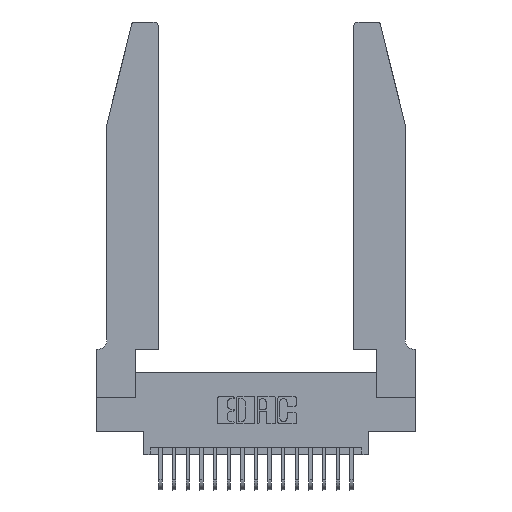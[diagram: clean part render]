
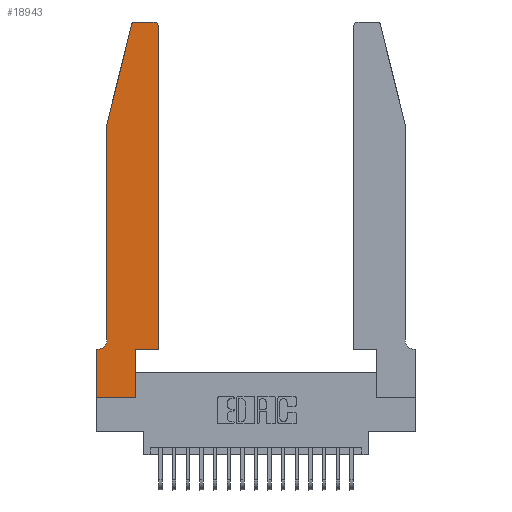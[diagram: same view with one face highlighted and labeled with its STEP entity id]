
A CAD part, top view. The second image highlights one B-rep face of the part: STEP entity #18943.
In plain terms, the highlighted planar face has unit normal (0, 0, 1).
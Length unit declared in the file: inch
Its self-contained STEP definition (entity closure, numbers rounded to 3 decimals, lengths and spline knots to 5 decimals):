
#37 = AXIS2_PLACEMENT_3D ( 'NONE', #13220, #3085, #14944 ) ;
#195 = ORIENTED_EDGE ( 'NONE', *, *, #10193, .T. ) ;
#387 = ORIENTED_EDGE ( 'NONE', *, *, #18961, .T. ) ;
#480 = CARTESIAN_POINT ( 'NONE',  ( 0.284, 2.75, 0.37 ) ) ;
#487 = DIRECTION ( 'NONE',  ( 1., 0., 0. ) ) ;
#775 = DIRECTION ( 'NONE',  ( 1., 0., 0. ) ) ;
#1053 = VERTEX_POINT ( 'NONE', #480 ) ;
#1071 = CARTESIAN_POINT ( 'NONE',  ( 0.4505, 0.35, 0.37 ) ) ;
#1951 = LINE ( 'NONE', #21206, #5494 ) ;
#1986 = VECTOR ( 'NONE', #10665, 39.37008 ) ;
#2110 = EDGE_LOOP ( 'NONE', ( #387, #195, #18907, #20903, #11278, #15937, #6031, #13395, #3044, #10007, #4897, #3687 ) ) ;
#2429 = VECTOR ( 'NONE', #4687, 39.37008 ) ;
#2494 = EDGE_CURVE ( 'NONE', #15002, #19544, #7154, .T. ) ;
#2525 = VERTEX_POINT ( 'NONE', #14175 ) ;
#2544 = CARTESIAN_POINT ( 'NONE',  ( 0., 0.35, 0.37 ) ) ;
#2557 = DIRECTION ( 'NONE',  ( 0., 0., 1. ) ) ;
#2631 = DIRECTION ( 'NONE',  ( -1., 0., 0. ) ) ;
#2947 = CARTESIAN_POINT ( 'NONE',  ( 0.0755, 0.35, 0.37 ) ) ;
#3044 = ORIENTED_EDGE ( 'NONE', *, *, #2494, .T. ) ;
#3047 = CARTESIAN_POINT ( 'NONE',  ( 0.0055, 0.35, 0.37 ) ) ;
#3085 = DIRECTION ( 'NONE',  ( 0., 0., -1. ) ) ;
#3164 = AXIS2_PLACEMENT_3D ( 'NONE', #20830, #10757, #487 ) ;
#3174 = CARTESIAN_POINT ( 'NONE',  ( 0.0755, 2., 0.37 ) ) ;
#3519 = EDGE_CURVE ( 'NONE', #15078, #15002, #1951, .T. ) ;
#3687 = ORIENTED_EDGE ( 'NONE', *, *, #5299, .T. ) ;
#4062 = VERTEX_POINT ( 'NONE', #18495 ) ;
#4203 = DIRECTION ( 'NONE',  ( 0., 1., 0. ) ) ;
#4465 = CARTESIAN_POINT ( 'NONE',  ( 0.4205, 2.75, 0.37 ) ) ;
#4687 = DIRECTION ( 'NONE',  ( -1., 0., 0. ) ) ;
#4728 = EDGE_CURVE ( 'NONE', #10207, #15078, #14430, .T. ) ;
#4827 = AXIS2_PLACEMENT_3D ( 'NONE', #21090, #11024, #775 ) ;
#4830 = CIRCLE ( 'NONE', #37, 0.07 ) ;
#4897 = ORIENTED_EDGE ( 'NONE', *, *, #21075, .T. ) ;
#4906 = LINE ( 'NONE', #12228, #13327 ) ;
#5299 = EDGE_CURVE ( 'NONE', #4062, #16967, #16251, .T. ) ;
#5494 = VECTOR ( 'NONE', #21252, 39.37008 ) ;
#5569 = EDGE_CURVE ( 'NONE', #7996, #10207, #15981, .T. ) ;
#6031 = ORIENTED_EDGE ( 'NONE', *, *, #4728, .T. ) ;
#6764 = DIRECTION ( 'NONE',  ( 0., -1., 0. ) ) ;
#6854 = VERTEX_POINT ( 'NONE', #18290 ) ;
#7154 = LINE ( 'NONE', #19578, #1986 ) ;
#7356 = LINE ( 'NONE', #9435, #20232 ) ;
#7603 = DIRECTION ( 'NONE',  ( -0.239, -0.971, 0. ) ) ;
#7996 = VERTEX_POINT ( 'NONE', #3047 ) ;
#9435 = CARTESIAN_POINT ( 'NONE',  ( 0.2605, 2.75, 0.37 ) ) ;
#9469 = CARTESIAN_POINT ( 'NONE',  ( 0., 0., 0.37 ) ) ;
#9618 = DIRECTION ( 'NONE',  ( 1., 0., 0. ) ) ;
#9681 = VECTOR ( 'NONE', #7603, 39.37008 ) ;
#10007 = ORIENTED_EDGE ( 'NONE', *, *, #13969, .T. ) ;
#10193 = EDGE_CURVE ( 'NONE', #1053, #16774, #18262, .T. ) ;
#10207 = VERTEX_POINT ( 'NONE', #2544 ) ;
#10665 = DIRECTION ( 'NONE',  ( 0., 1., 0. ) ) ;
#10685 = CARTESIAN_POINT ( 'NONE',  ( 0.25487, 2.72718, 0.37 ) ) ;
#10757 = DIRECTION ( 'NONE',  ( 0., 0., 1. ) ) ;
#11024 = DIRECTION ( 'NONE',  ( 0., 0., 1. ) ) ;
#11278 = ORIENTED_EDGE ( 'NONE', *, *, #15303, .T. ) ;
#12228 = CARTESIAN_POINT ( 'NONE',  ( 0.4505, 0.35, 0.37 ) ) ;
#12495 = CARTESIAN_POINT ( 'NONE',  ( 0., 0., 0.37 ) ) ;
#12704 = PLANE ( 'NONE',  #20468 ) ;
#13053 = CARTESIAN_POINT ( 'NONE',  ( 0.2865, 0.35, 0.37 ) ) ;
#13220 = CARTESIAN_POINT ( 'NONE',  ( 0.0055, 0.42, 0.37 ) ) ;
#13281 = CARTESIAN_POINT ( 'NONE',  ( 0.0755, 0.42, 0.37 ) ) ;
#13327 = VECTOR ( 'NONE', #4203, 39.37008 ) ;
#13395 = ORIENTED_EDGE ( 'NONE', *, *, #3519, .T. ) ;
#13444 = EDGE_CURVE ( 'NONE', #16774, #2525, #15205, .T. ) ;
#13512 = LINE ( 'NONE', #3174, #21902 ) ;
#13969 = EDGE_CURVE ( 'NONE', #19544, #6854, #14118, .T. ) ;
#14118 = LINE ( 'NONE', #1071, #21966 ) ;
#14175 = CARTESIAN_POINT ( 'NONE',  ( 0.0755, 2., 0.37 ) ) ;
#14430 = LINE ( 'NONE', #9469, #18924 ) ;
#14432 = DIRECTION ( 'NONE',  ( 1., 0., 0. ) ) ;
#14752 = EDGE_CURVE ( 'NONE', #2525, #20800, #13512, .T. ) ;
#14944 = DIRECTION ( 'NONE',  ( -1., 0., 0. ) ) ;
#15002 = VERTEX_POINT ( 'NONE', #17534 ) ;
#15078 = VERTEX_POINT ( 'NONE', #12495 ) ;
#15205 = LINE ( 'NONE', #19207, #9681 ) ;
#15303 = EDGE_CURVE ( 'NONE', #20800, #7996, #4830, .T. ) ;
#15937 = ORIENTED_EDGE ( 'NONE', *, *, #5569, .T. ) ;
#15981 = LINE ( 'NONE', #2947, #2429 ) ;
#16058 = CARTESIAN_POINT ( 'NONE',  ( 0., 0.35, 0.37 ) ) ;
#16251 = CIRCLE ( 'NONE', #3164, 0.03 ) ;
#16774 = VERTEX_POINT ( 'NONE', #10685 ) ;
#16824 = FACE_OUTER_BOUND ( 'NONE', #2110, .T. ) ;
#16967 = VERTEX_POINT ( 'NONE', #4465 ) ;
#17534 = CARTESIAN_POINT ( 'NONE',  ( 0.2865, 0., 0.37 ) ) ;
#18262 = CIRCLE ( 'NONE', #4827, 0.03 ) ;
#18290 = CARTESIAN_POINT ( 'NONE',  ( 0.4505, 0.35, 0.37 ) ) ;
#18495 = CARTESIAN_POINT ( 'NONE',  ( 0.4505, 2.72, 0.37 ) ) ;
#18907 = ORIENTED_EDGE ( 'NONE', *, *, #13444, .T. ) ;
#18924 = VECTOR ( 'NONE', #21211, 39.37008 ) ;
#18943 = ADVANCED_FACE ( 'NONE', ( #16824 ), #12704, .T. ) ;
#18961 = EDGE_CURVE ( 'NONE', #16967, #1053, #7356, .T. ) ;
#19207 = CARTESIAN_POINT ( 'NONE',  ( 0.0755, 2., 0.37 ) ) ;
#19544 = VERTEX_POINT ( 'NONE', #13053 ) ;
#19578 = CARTESIAN_POINT ( 'NONE',  ( 0.2865, 0.35, 0.37 ) ) ;
#20232 = VECTOR ( 'NONE', #2631, 39.37008 ) ;
#20468 = AXIS2_PLACEMENT_3D ( 'NONE', #16058, #2557, #14432 ) ;
#20800 = VERTEX_POINT ( 'NONE', #13281 ) ;
#20830 = CARTESIAN_POINT ( 'NONE',  ( 0.4205, 2.72, 0.37 ) ) ;
#20903 = ORIENTED_EDGE ( 'NONE', *, *, #14752, .T. ) ;
#21075 = EDGE_CURVE ( 'NONE', #6854, #4062, #4906, .T. ) ;
#21090 = CARTESIAN_POINT ( 'NONE',  ( 0.284, 2.72, 0.37 ) ) ;
#21206 = CARTESIAN_POINT ( 'NONE',  ( 0., 0., 0.37 ) ) ;
#21211 = DIRECTION ( 'NONE',  ( 0., -1., 0. ) ) ;
#21252 = DIRECTION ( 'NONE',  ( 1., 0., 0. ) ) ;
#21902 = VECTOR ( 'NONE', #6764, 39.37008 ) ;
#21966 = VECTOR ( 'NONE', #9618, 39.37008 ) ;
